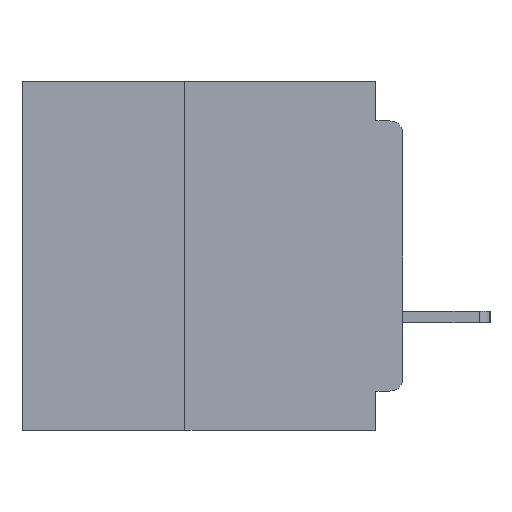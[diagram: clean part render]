
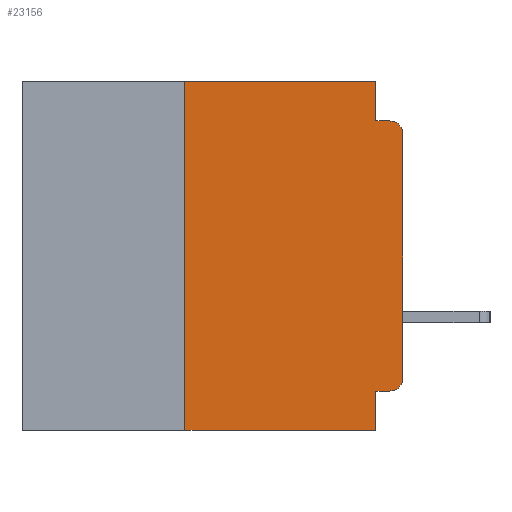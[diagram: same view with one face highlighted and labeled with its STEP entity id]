
A CAD part, left-side view. The second image highlights one B-rep face of the part: STEP entity #23156.
In plain terms, the highlighted planar face has unit normal (-1, 0, 0).
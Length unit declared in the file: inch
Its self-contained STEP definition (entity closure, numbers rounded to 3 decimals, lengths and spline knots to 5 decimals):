
#563 = EDGE_CURVE ( 'NONE', #17119, #18367, #1701, .T. ) ;
#777 = EDGE_CURVE ( 'NONE', #14469, #33047, #11201, .T. ) ;
#1701 = LINE ( 'NONE', #30537, #22716 ) ;
#1825 = EDGE_CURVE ( 'NONE', #11078, #14469, #7877, .T. ) ;
#2438 = ORIENTED_EDGE ( 'NONE', *, *, #563, .F. ) ;
#3292 = VECTOR ( 'NONE', #23386, 39.37008 ) ;
#3955 = CARTESIAN_POINT ( 'NONE',  ( 0., 0.015, -0.06 ) ) ;
#3975 = VECTOR ( 'NONE', #21214, 39.37008 ) ;
#4134 = ORIENTED_EDGE ( 'NONE', *, *, #23381, .T. ) ;
#4155 = PLANE ( 'NONE',  #33453 ) ;
#4302 = EDGE_LOOP ( 'NONE', ( #10666, #17985, #19970, #4885, #11498, #2438, #23110, #32614, #10460, #4134 ) ) ;
#4885 = ORIENTED_EDGE ( 'NONE', *, *, #31778, .F. ) ;
#6762 = DIRECTION ( 'NONE',  ( 0., 0., -1. ) ) ;
#6949 = DIRECTION ( 'NONE',  ( 1., 0., 0. ) ) ;
#7323 = DIRECTION ( 'NONE',  ( 0., -1., 0. ) ) ;
#7611 = DIRECTION ( 'NONE',  ( 0., 0., -1. ) ) ;
#7877 = LINE ( 'NONE', #12730, #14324 ) ;
#9407 = CIRCLE ( 'NONE', #11080, 0.015 ) ;
#9511 = VECTOR ( 'NONE', #7611, 39.37008 ) ;
#9830 = CIRCLE ( 'NONE', #32065, 0.015 ) ;
#9843 = FACE_OUTER_BOUND ( 'NONE', #4302, .T. ) ;
#10460 = ORIENTED_EDGE ( 'NONE', *, *, #1825, .F. ) ;
#10516 = VECTOR ( 'NONE', #7323, 39.37008 ) ;
#10666 = ORIENTED_EDGE ( 'NONE', *, *, #32119, .T. ) ;
#10698 = CARTESIAN_POINT ( 'NONE',  ( 0., 0.031, -0.4 ) ) ;
#10873 = DIRECTION ( 'NONE',  ( 0., 0., -1. ) ) ;
#11078 = VERTEX_POINT ( 'NONE', #27847 ) ;
#11080 = AXIS2_PLACEMENT_3D ( 'NONE', #13424, #32237, #16145 ) ;
#11088 = CARTESIAN_POINT ( 'NONE',  ( 0., 0.031, -0.045 ) ) ;
#11201 = LINE ( 'NONE', #10698, #9511 ) ;
#11498 = ORIENTED_EDGE ( 'NONE', *, *, #20833, .F. ) ;
#12569 = DIRECTION ( 'NONE',  ( 0., 0., 1. ) ) ;
#12730 = CARTESIAN_POINT ( 'NONE',  ( 0., 0., -0.355 ) ) ;
#12734 = VECTOR ( 'NONE', #23325, 39.37008 ) ;
#13046 = CARTESIAN_POINT ( 'NONE',  ( 0., 0., -0.06 ) ) ;
#13424 = CARTESIAN_POINT ( 'NONE',  ( 0., 0.015, -0.34 ) ) ;
#14324 = VECTOR ( 'NONE', #25629, 39.37008 ) ;
#14469 = VERTEX_POINT ( 'NONE', #35083 ) ;
#15088 = CARTESIAN_POINT ( 'NONE',  ( 0., 0.437, 0. ) ) ;
#15443 = EDGE_CURVE ( 'NONE', #29251, #22441, #9830, .T. ) ;
#15866 = EDGE_CURVE ( 'NONE', #17119, #33047, #25085, .T. ) ;
#15961 = CARTESIAN_POINT ( 'NONE',  ( 0., 0.25, -0.4 ) ) ;
#16145 = DIRECTION ( 'NONE',  ( 0., 0., -1. ) ) ;
#16524 = CARTESIAN_POINT ( 'NONE',  ( 0., 0.031, -0.4 ) ) ;
#16638 = VERTEX_POINT ( 'NONE', #11088 ) ;
#17054 = CARTESIAN_POINT ( 'NONE',  ( 0., 0.015, -0.045 ) ) ;
#17119 = VERTEX_POINT ( 'NONE', #15961 ) ;
#17445 = LINE ( 'NONE', #32468, #31719 ) ;
#17985 = ORIENTED_EDGE ( 'NONE', *, *, #15443, .T. ) ;
#18367 = VERTEX_POINT ( 'NONE', #29278 ) ;
#18501 = CARTESIAN_POINT ( 'NONE',  ( 0., 0.437, 0. ) ) ;
#19088 = CARTESIAN_POINT ( 'NONE',  ( 0., 0., -0.34 ) ) ;
#19970 = ORIENTED_EDGE ( 'NONE', *, *, #32800, .F. ) ;
#20681 = CARTESIAN_POINT ( 'NONE',  ( 0., 0.437, -0.4 ) ) ;
#20833 = EDGE_CURVE ( 'NONE', #18367, #31799, #25732, .T. ) ;
#20938 = CARTESIAN_POINT ( 'NONE',  ( 0., 0., -0.045 ) ) ;
#20996 = VERTEX_POINT ( 'NONE', #19088 ) ;
#21214 = DIRECTION ( 'NONE',  ( 0., -1., 0. ) ) ;
#22441 = VERTEX_POINT ( 'NONE', #17054 ) ;
#22716 = VECTOR ( 'NONE', #12569, 39.37008 ) ;
#23071 = DIRECTION ( 'NONE',  ( -1., 0., 0. ) ) ;
#23110 = ORIENTED_EDGE ( 'NONE', *, *, #15866, .T. ) ;
#23156 = ADVANCED_FACE ( 'NONE', ( #9843 ), #4155, .F. ) ;
#23325 = DIRECTION ( 'NONE',  ( 0., 0., 1. ) ) ;
#23381 = EDGE_CURVE ( 'NONE', #11078, #20996, #9407, .T. ) ;
#23386 = DIRECTION ( 'NONE',  ( 0., -1., 0. ) ) ;
#25085 = LINE ( 'NONE', #20681, #3292 ) ;
#25629 = DIRECTION ( 'NONE',  ( 0., 1., 0. ) ) ;
#25732 = LINE ( 'NONE', #18501, #3975 ) ;
#25798 = LINE ( 'NONE', #20938, #10516 ) ;
#25955 = DIRECTION ( 'NONE',  ( 0., 0., -1. ) ) ;
#27847 = CARTESIAN_POINT ( 'NONE',  ( 0., 0.015, -0.355 ) ) ;
#29251 = VERTEX_POINT ( 'NONE', #13046 ) ;
#29278 = CARTESIAN_POINT ( 'NONE',  ( 0., 0.25, 0. ) ) ;
#30537 = CARTESIAN_POINT ( 'NONE',  ( 0., 0.25, -0.4 ) ) ;
#31160 = CARTESIAN_POINT ( 'NONE',  ( 0., 0., 0. ) ) ;
#31719 = VECTOR ( 'NONE', #10873, 39.37008 ) ;
#31778 = EDGE_CURVE ( 'NONE', #31799, #16638, #17445, .T. ) ;
#31799 = VERTEX_POINT ( 'NONE', #32578 ) ;
#32065 = AXIS2_PLACEMENT_3D ( 'NONE', #3955, #23071, #6762 ) ;
#32119 = EDGE_CURVE ( 'NONE', #20996, #29251, #34223, .T. ) ;
#32237 = DIRECTION ( 'NONE',  ( -1., 0., 0. ) ) ;
#32468 = CARTESIAN_POINT ( 'NONE',  ( 0., 0.031, 0. ) ) ;
#32578 = CARTESIAN_POINT ( 'NONE',  ( 0., 0.031, 0. ) ) ;
#32614 = ORIENTED_EDGE ( 'NONE', *, *, #777, .F. ) ;
#32800 = EDGE_CURVE ( 'NONE', #16638, #22441, #25798, .T. ) ;
#33047 = VERTEX_POINT ( 'NONE', #16524 ) ;
#33453 = AXIS2_PLACEMENT_3D ( 'NONE', #15088, #6949, #25955 ) ;
#34223 = LINE ( 'NONE', #31160, #12734 ) ;
#35083 = CARTESIAN_POINT ( 'NONE',  ( 0., 0.031, -0.355 ) ) ;
